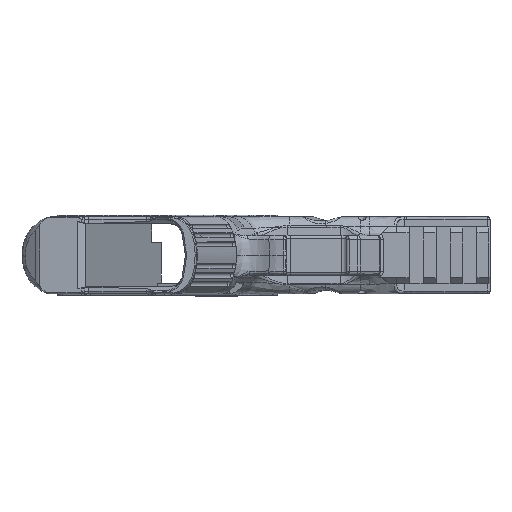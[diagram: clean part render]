
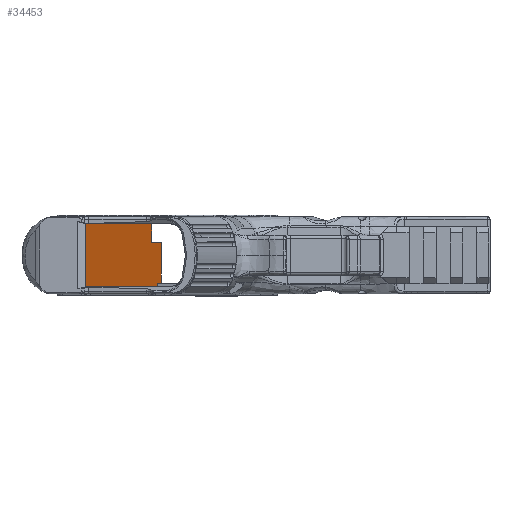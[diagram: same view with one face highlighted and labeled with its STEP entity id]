
A CAD part, front view. The second image highlights one B-rep face of the part: STEP entity #34453.
In plain terms, the highlighted planar face has unit normal (0.951, -0.309, 0).
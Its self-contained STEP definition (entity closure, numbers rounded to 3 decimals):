
#1515=LINE('',#51601,#4072);
#1521=LINE('',#51613,#4078);
#1522=LINE('',#51615,#4079);
#1523=LINE('',#51617,#4080);
#1524=LINE('',#51619,#4081);
#1525=LINE('',#51621,#4082);
#1526=LINE('',#51623,#4083);
#1527=LINE('',#51624,#4084);
#4072=VECTOR('',#38430,10.);
#4078=VECTOR('',#38438,10.);
#4079=VECTOR('',#38439,10.);
#4080=VECTOR('',#38440,10.);
#4081=VECTOR('',#38441,10.);
#4082=VECTOR('',#38442,10.);
#4083=VECTOR('',#38443,10.);
#4084=VECTOR('',#38444,10.);
#7560=PLANE('',#36488);
#8614=FACE_OUTER_BOUND('',#10622,.T.);
#10622=EDGE_LOOP('',(#23496,#23497,#23498,#23499,#23500,#23501,#23502,#23503));
#14225=VERTEX_POINT('',#51599);
#14226=VERTEX_POINT('',#51600);
#14231=VERTEX_POINT('',#51612);
#14232=VERTEX_POINT('',#51614);
#14233=VERTEX_POINT('',#51616);
#14234=VERTEX_POINT('',#51618);
#14235=VERTEX_POINT('',#51620);
#14236=VERTEX_POINT('',#51622);
#17839=EDGE_CURVE('',#14225,#14226,#1515,.T.);
#17845=EDGE_CURVE('',#14226,#14231,#1521,.T.);
#17846=EDGE_CURVE('',#14232,#14231,#1522,.T.);
#17847=EDGE_CURVE('',#14233,#14232,#1523,.T.);
#17848=EDGE_CURVE('',#14234,#14233,#1524,.T.);
#17849=EDGE_CURVE('',#14235,#14234,#1525,.T.);
#17850=EDGE_CURVE('',#14236,#14235,#1526,.T.);
#17851=EDGE_CURVE('',#14236,#14225,#1527,.T.);
#23496=ORIENTED_EDGE('',*,*,#17839,.T.);
#23497=ORIENTED_EDGE('',*,*,#17845,.T.);
#23498=ORIENTED_EDGE('',*,*,#17846,.F.);
#23499=ORIENTED_EDGE('',*,*,#17847,.F.);
#23500=ORIENTED_EDGE('',*,*,#17848,.F.);
#23501=ORIENTED_EDGE('',*,*,#17849,.F.);
#23502=ORIENTED_EDGE('',*,*,#17850,.F.);
#23503=ORIENTED_EDGE('',*,*,#17851,.T.);
#34453=ADVANCED_FACE('',(#8614),#7560,.F.);
#36488=AXIS2_PLACEMENT_3D('',#51611,#38436,#38437);
#38430=DIRECTION('',(0.,0.,-1.));
#38436=DIRECTION('center_axis',(-0.951,0.309,0.));
#38437=DIRECTION('ref_axis',(0.,0.,
1.));
#38438=DIRECTION('',(0.309,0.951,0.));
#38439=DIRECTION('',(0.,0.,-1.));
#38440=DIRECTION('',(-0.309,-0.951,0.));
#38441=DIRECTION('',(0.,0.,-1.));
#38442=DIRECTION('',(0.309,0.951,0.));
#38443=DIRECTION('',(0.,0.,-1.));
#38444=DIRECTION('',(-0.309,-0.951,0.));
#51599=CARTESIAN_POINT('',(5.324,-88.495,11.75));
#51600=CARTESIAN_POINT('',(5.324,-88.495,-11.75));
#51601=CARTESIAN_POINT('',(5.324,-88.495,-14.607));
#51611=CARTESIAN_POINT('Origin',(2.312,-97.765,-11.75));
#51612=CARTESIAN_POINT('',(32.169,-5.875,-11.75));
#51613=CARTESIAN_POINT('',(2.312,-97.765,-11.75));
#51614=CARTESIAN_POINT('',(32.169,-5.875,-10.375));
#51615=CARTESIAN_POINT('',(32.169,-5.875,-5.875));
#51616=CARTESIAN_POINT('',(33.591,-1.5,-10.375));
#51617=CARTESIAN_POINT('',(17.241,-51.82,-10.375));
#51618=CARTESIAN_POINT('',(33.591,-1.5,4.75));
#51619=CARTESIAN_POINT('',(33.591,-1.5,-5.875));
#51620=CARTESIAN_POINT('',(30.049,-12.4,4.75));
#51621=CARTESIAN_POINT('',(18.86,-46.836,4.75));
#51622=CARTESIAN_POINT('',(30.049,-12.4,11.75));
#51623=CARTESIAN_POINT('',(30.049,-12.4,2.982));
#51624=CARTESIAN_POINT('',(2.312,-97.765,11.75));
